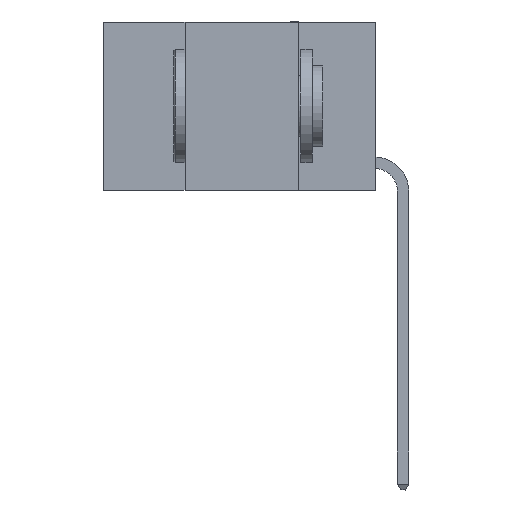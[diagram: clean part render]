
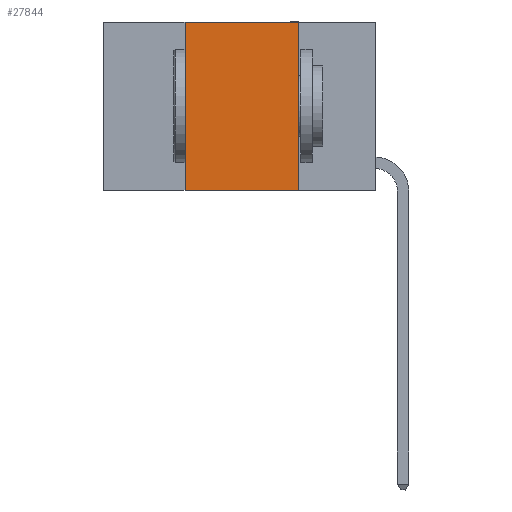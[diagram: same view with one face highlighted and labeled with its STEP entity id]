
A CAD part, left-side view. The second image highlights one B-rep face of the part: STEP entity #27844.
In plain terms, the highlighted planar face has unit normal (-1, 0, 0).
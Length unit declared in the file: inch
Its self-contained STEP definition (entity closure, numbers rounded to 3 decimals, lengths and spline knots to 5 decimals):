
#1044 = DIRECTION ( 'NONE',  ( 0., 0., 1. ) ) ;
#1135 = CARTESIAN_POINT ( 'NONE',  ( 0., 0.6, 0. ) ) ;
#5066 = VERTEX_POINT ( 'NONE', #13465 ) ;
#5187 = LINE ( 'NONE', #1135, #30398 ) ;
#5778 = VERTEX_POINT ( 'NONE', #11541 ) ;
#6028 = DIRECTION ( 'NONE',  ( 0., -1., 0. ) ) ;
#6219 = EDGE_CURVE ( 'NONE', #5778, #30396, #10607, .T. ) ;
#8053 = EDGE_LOOP ( 'NONE', ( #17592, #13032, #12842, #28180 ) ) ;
#9030 = DIRECTION ( 'NONE',  ( 1., 0., 0. ) ) ;
#10595 = DIRECTION ( 'NONE',  ( 0., 0., -1. ) ) ;
#10607 = LINE ( 'NONE', #24962, #16150 ) ;
#11295 = PLANE ( 'NONE',  #14761 ) ;
#11541 = CARTESIAN_POINT ( 'NONE',  ( 0., 0.42, -0.37 ) ) ;
#12247 = FACE_OUTER_BOUND ( 'NONE', #8053, .T. ) ;
#12277 = EDGE_CURVE ( 'NONE', #5066, #26619, #5187, .T. ) ;
#12660 = LINE ( 'NONE', #19999, #30092 ) ;
#12834 = CARTESIAN_POINT ( 'NONE',  ( 0., 0.17, -0.37 ) ) ;
#12842 = ORIENTED_EDGE ( 'NONE', *, *, #17443, .F. ) ;
#13032 = ORIENTED_EDGE ( 'NONE', *, *, #12277, .F. ) ;
#13465 = CARTESIAN_POINT ( 'NONE',  ( 0., 0.42, 0. ) ) ;
#14761 = AXIS2_PLACEMENT_3D ( 'NONE', #23180, #9030, #25568 ) ;
#16150 = VECTOR ( 'NONE', #6028, 39.37008 ) ;
#17443 = EDGE_CURVE ( 'NONE', #5778, #5066, #30355, .T. ) ;
#17592 = ORIENTED_EDGE ( 'NONE', *, *, #23119, .F. ) ;
#17787 = DIRECTION ( 'NONE',  ( 0., -1., 0. ) ) ;
#18465 = VECTOR ( 'NONE', #1044, 39.37008 ) ;
#19999 = CARTESIAN_POINT ( 'NONE',  ( 0., 0.17, 0. ) ) ;
#23119 = EDGE_CURVE ( 'NONE', #26619, #30396, #12660, .T. ) ;
#23180 = CARTESIAN_POINT ( 'NONE',  ( 0., 0.6, 0. ) ) ;
#23356 = CARTESIAN_POINT ( 'NONE',  ( 0., 0.17, 0. ) ) ;
#24962 = CARTESIAN_POINT ( 'NONE',  ( 0., 0.6, -0.37 ) ) ;
#25568 = DIRECTION ( 'NONE',  ( 0., 0., -1. ) ) ;
#26619 = VERTEX_POINT ( 'NONE', #23356 ) ;
#27844 = ADVANCED_FACE ( 'NONE', ( #12247 ), #11295, .F. ) ;
#28180 = ORIENTED_EDGE ( 'NONE', *, *, #6219, .T. ) ;
#29542 = CARTESIAN_POINT ( 'NONE',  ( 0., 0.42, 0. ) ) ;
#30092 = VECTOR ( 'NONE', #10595, 39.37008 ) ;
#30355 = LINE ( 'NONE', #29542, #18465 ) ;
#30396 = VERTEX_POINT ( 'NONE', #12834 ) ;
#30398 = VECTOR ( 'NONE', #17787, 39.37008 ) ;
